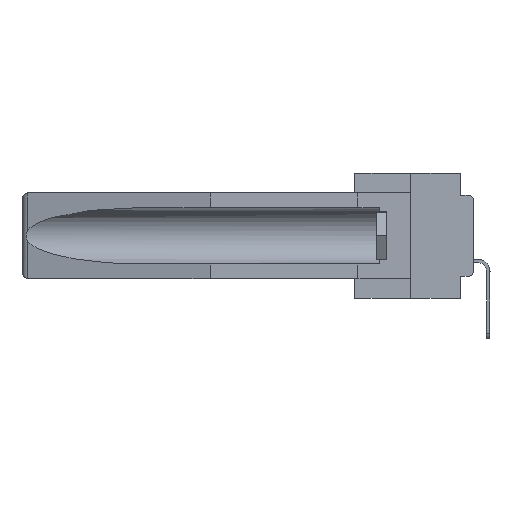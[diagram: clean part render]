
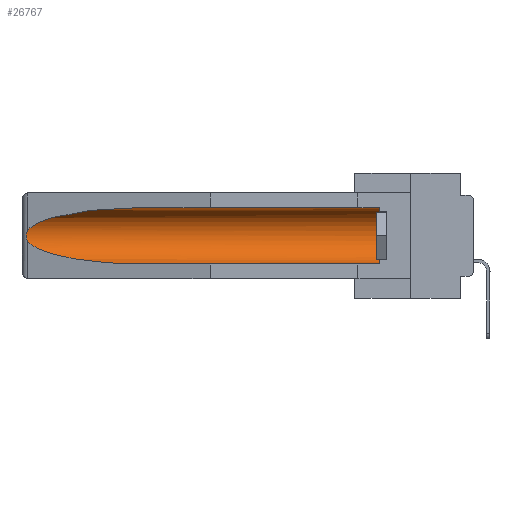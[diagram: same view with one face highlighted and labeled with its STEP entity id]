
A CAD part, left-side view. The second image highlights one B-rep face of the part: STEP entity #26767.
In plain terms, the highlighted cylindrical face has radius 2.857 mm (diameter 5.715 mm), a partial arc.
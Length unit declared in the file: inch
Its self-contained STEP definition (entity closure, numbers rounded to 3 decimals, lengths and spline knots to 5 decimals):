
#553 = B_SPLINE_CURVE_WITH_KNOTS ( 'NONE', 3,
 ( #24084, #15033, #10525, #1047, #12777, #19834, #22241, #29022, #17432, #26618 ),
 .UNSPECIFIED., .F., .F.,
 ( 4, 2, 2, 2, 4 ),
 ( 0., 0.00029, 0.00058, 0.00087, 0.00117 ),
 .UNSPECIFIED. ) ;
#1047 = CARTESIAN_POINT ( 'NONE',  ( 0.2673, 1.5327, -0.16383 ) ) ;
#1804 = VECTOR ( 'NONE', #28373, 39.37008 ) ;
#2236 = CARTESIAN_POINT ( 'NONE',  ( 0.155, 1.07973, -0.284 ) ) ;
#3020 = VERTEX_POINT ( 'NONE', #6291 ) ;
#3070 = CARTESIAN_POINT ( 'NONE',  ( 0.155, 0.126, -0.284 ) ) ;
#3102 = AXIS2_PLACEMENT_3D ( 'NONE', #28376, #19196, #7605 ) ;
#3645 =( BOUNDED_CURVE ( )  B_SPLINE_CURVE ( 3, ( #17929, #13431, #24720, #6811 ),
 .UNSPECIFIED., .F., .T. ) 
 B_SPLINE_CURVE_WITH_KNOTS ( ( 4, 4 ),
 ( 4.71239, 6.08839 ),
 .UNSPECIFIED. ) 
 CURVE ( )  GEOMETRIC_REPRESENTATION_ITEM ( )  RATIONAL_B_SPLINE_CURVE ( ( 1., 0.848, 0.848, 1. ) ) 
 REPRESENTATION_ITEM ( '' )  );
#3684 = CARTESIAN_POINT ( 'NONE',  ( 0.26537, 1.52718, -0.14972 ) ) ;
#3880 = EDGE_CURVE ( 'NONE', #22293, #13194, #22026, .T. ) ;
#5200 = CYLINDRICAL_SURFACE ( 'NONE', #3102, 0.1125 ) ;
#6291 = CARTESIAN_POINT ( 'NONE',  ( 0.155, 1.07973, -0.059 ) ) ;
#6572 = ORIENTED_EDGE ( 'NONE', *, *, #10688, .T. ) ;
#6701 = LINE ( 'NONE', #26256, #1804 ) ;
#6811 = CARTESIAN_POINT ( 'NONE',  ( 0.26537, 1.52718, -0.14972 ) ) ;
#6902 = CARTESIAN_POINT ( 'NONE',  ( 0.21114, 1.30732, -0.284 ) ) ;
#7477 = ORIENTED_EDGE ( 'NONE', *, *, #25459, .T. ) ;
#7566 = EDGE_CURVE ( 'NONE', #22293, #12904, #9502, .T. ) ;
#7605 = DIRECTION ( 'NONE',  ( 0., 0., 1. ) ) ;
#8082 = ORIENTED_EDGE ( 'NONE', *, *, #3880, .F. ) ;
#9136 = EDGE_CURVE ( 'NONE', #12904, #3020, #6701, .T. ) ;
#9502 = CIRCLE ( 'NONE', #24347, 0.1125 ) ;
#10006 = FACE_OUTER_BOUND ( 'NONE', #24986, .T. ) ;
#10525 = CARTESIAN_POINT ( 'NONE',  ( 0.26654, 1.53092, -0.15636 ) ) ;
#10688 = EDGE_CURVE ( 'NONE', #19345, #25183, #553, .T. ) ;
#10898 = ORIENTED_EDGE ( 'NONE', *, *, #7566, .T. ) ;
#11046 = ORIENTED_EDGE ( 'NONE', *, *, #27124, .T. ) ;
#12777 = CARTESIAN_POINT ( 'NONE',  ( 0.2675, 1.53308, -0.16763 ) ) ;
#12904 = VERTEX_POINT ( 'NONE', #13585 ) ;
#13194 = VERTEX_POINT ( 'NONE', #16910 ) ;
#13431 = CARTESIAN_POINT ( 'NONE',  ( 0.21114, 1.30732, -0.059 ) ) ;
#13585 = CARTESIAN_POINT ( 'NONE',  ( 0.155, 0.126, -0.059 ) ) ;
#15033 = CARTESIAN_POINT ( 'NONE',  ( 0.26597, 1.52961, -0.15275 ) ) ;
#16910 = CARTESIAN_POINT ( 'NONE',  ( 0.155, 1.07973, -0.284 ) ) ;
#17432 = CARTESIAN_POINT ( 'NONE',  ( 0.26597, 1.5296, -0.19026 ) ) ;
#17646 = CARTESIAN_POINT ( 'NONE',  ( 0.155, -0.30754, -0.284 ) ) ;
#17920 = CARTESIAN_POINT ( 'NONE',  ( 0.155, 0.126, -0.1715 ) ) ;
#17929 = CARTESIAN_POINT ( 'NONE',  ( 0.155, 1.07973, -0.059 ) ) ;
#18242 = DIRECTION ( 'NONE',  ( 0., 0., 1. ) ) ;
#19196 = DIRECTION ( 'NONE',  ( 0., 1., 0. ) ) ;
#19345 = VERTEX_POINT ( 'NONE', #3684 ) ;
#19834 = CARTESIAN_POINT ( 'NONE',  ( 0.2675, 1.53308, -0.17534 ) ) ;
#20605 = CARTESIAN_POINT ( 'NONE',  ( 0.26537, 1.52718, -0.19328 ) ) ;
#20686 = ORIENTED_EDGE ( 'NONE', *, *, #9136, .T. ) ;
#21815 = CARTESIAN_POINT ( 'NONE',  ( 0.26537, 1.52718, -0.19328 ) ) ;
#22026 = LINE ( 'NONE', #17646, #29510 ) ;
#22172 = DIRECTION ( 'NONE',  ( 0., 1., 0. ) ) ;
#22241 = CARTESIAN_POINT ( 'NONE',  ( 0.2673, 1.53269, -0.17917 ) ) ;
#22293 = VERTEX_POINT ( 'NONE', #3070 ) ;
#22602 = DIRECTION ( 'NONE',  ( 0., -1., 0. ) ) ;
#24084 = CARTESIAN_POINT ( 'NONE',  ( 0.26537, 1.52718, -0.14972 ) ) ;
#24347 = AXIS2_PLACEMENT_3D ( 'NONE', #17920, #22602, #18242 ) ;
#24720 = CARTESIAN_POINT ( 'NONE',  ( 0.25451, 1.48313, -0.09465 ) ) ;
#24986 = EDGE_LOOP ( 'NONE', ( #11046, #6572, #7477, #8082, #10898, #20686 ) ) ;
#25183 = VERTEX_POINT ( 'NONE', #21815 ) ;
#25459 = EDGE_CURVE ( 'NONE', #25183, #13194, #27297, .T. ) ;
#25730 = CARTESIAN_POINT ( 'NONE',  ( 0.25451, 1.48313, -0.24835 ) ) ;
#26256 = CARTESIAN_POINT ( 'NONE',  ( 0.155, -0.30754, -0.059 ) ) ;
#26618 = CARTESIAN_POINT ( 'NONE',  ( 0.26537, 1.52718, -0.19328 ) ) ;
#26767 = ADVANCED_FACE ( 'NONE', ( #10006 ), #5200, .F. ) ;
#27124 = EDGE_CURVE ( 'NONE', #3020, #19345, #3645, .T. ) ;
#27297 =( BOUNDED_CURVE ( )  B_SPLINE_CURVE ( 3, ( #20605, #25730, #6902, #2236 ),
 .UNSPECIFIED., .F., .F. ) 
 B_SPLINE_CURVE_WITH_KNOTS ( ( 4, 4 ),
 ( 0.1948, 1.5708 ),
 .UNSPECIFIED. ) 
 CURVE ( )  GEOMETRIC_REPRESENTATION_ITEM ( )  RATIONAL_B_SPLINE_CURVE ( ( 1., 0.848, 0.848, 1. ) ) 
 REPRESENTATION_ITEM ( '' )  );
#28373 = DIRECTION ( 'NONE',  ( 0., 1., 0. ) ) ;
#28376 = CARTESIAN_POINT ( 'NONE',  ( 0.155, -0.30754, -0.1715 ) ) ;
#29022 = CARTESIAN_POINT ( 'NONE',  ( 0.26655, 1.53094, -0.18657 ) ) ;
#29510 = VECTOR ( 'NONE', #22172, 39.37008 ) ;
